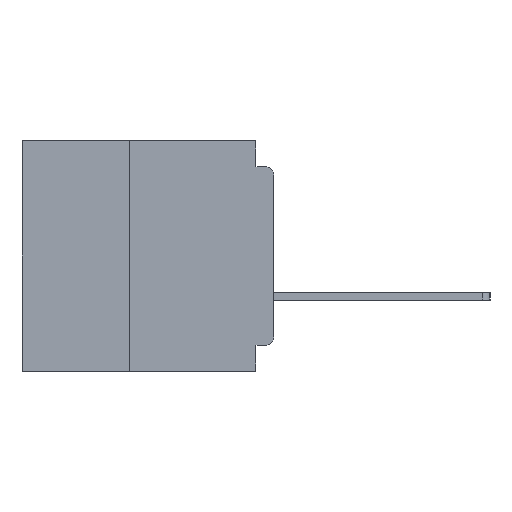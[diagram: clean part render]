
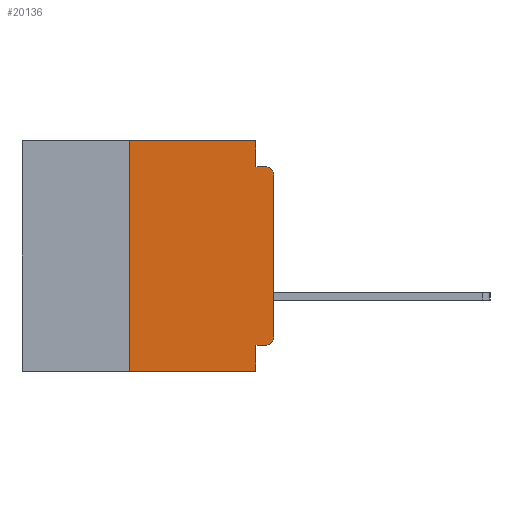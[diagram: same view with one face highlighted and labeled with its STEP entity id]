
A CAD part, left-side view. The second image highlights one B-rep face of the part: STEP entity #20136.
In plain terms, the highlighted planar face has unit normal (-1, 0, 0).
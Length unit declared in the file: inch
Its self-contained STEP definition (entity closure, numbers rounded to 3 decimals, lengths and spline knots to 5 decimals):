
#938 = ORIENTED_EDGE ( 'NONE', *, *, #48348, .F. ) ;
#1005 = VECTOR ( 'NONE', #35421, 39.37008 ) ;
#1330 = CARTESIAN_POINT ( 'NONE',  ( 0., 0.25, -0.4 ) ) ;
#1773 = VECTOR ( 'NONE', #25960, 39.37008 ) ;
#2149 = CIRCLE ( 'NONE', #40558, 0.015 ) ;
#2288 = DIRECTION ( 'NONE',  ( 0., -1., 0. ) ) ;
#2367 = VECTOR ( 'NONE', #25883, 39.37008 ) ;
#3299 = CARTESIAN_POINT ( 'NONE',  ( 0., 0.015, -0.045 ) ) ;
#5212 = ORIENTED_EDGE ( 'NONE', *, *, #49112, .T. ) ;
#5920 = VERTEX_POINT ( 'NONE', #15043 ) ;
#6289 = CARTESIAN_POINT ( 'NONE',  ( 0., 0., -0.355 ) ) ;
#7400 = CARTESIAN_POINT ( 'NONE',  ( 0., 0.015, -0.06 ) ) ;
#7617 = ORIENTED_EDGE ( 'NONE', *, *, #35024, .T. ) ;
#8090 = CARTESIAN_POINT ( 'NONE',  ( 0., 0.031, -0.355 ) ) ;
#8459 = VECTOR ( 'NONE', #44813, 39.37008 ) ;
#8874 = CARTESIAN_POINT ( 'NONE',  ( 0., 0.015, -0.34 ) ) ;
#9425 = VERTEX_POINT ( 'NONE', #21818 ) ;
#9551 = CARTESIAN_POINT ( 'NONE',  ( 0., 0.437, -0.4 ) ) ;
#10099 = CARTESIAN_POINT ( 'NONE',  ( 0., 0.437, 0. ) ) ;
#10802 = VECTOR ( 'NONE', #46721, 39.37008 ) ;
#11358 = DIRECTION ( 'NONE',  ( 0., 0., -1. ) ) ;
#11431 = LINE ( 'NONE', #39141, #1005 ) ;
#11525 = CARTESIAN_POINT ( 'NONE',  ( 0., 0.031, -0.4 ) ) ;
#12788 = CARTESIAN_POINT ( 'NONE',  ( 0., 0.031, 0. ) ) ;
#12807 = LINE ( 'NONE', #37500, #2367 ) ;
#12830 = DIRECTION ( 'NONE',  ( 0., 0., -1. ) ) ;
#14056 = DIRECTION ( 'NONE',  ( 0., 0., -1. ) ) ;
#15043 = CARTESIAN_POINT ( 'NONE',  ( 0., 0.031, -0.4 ) ) ;
#15621 = CIRCLE ( 'NONE', #40229, 0.015 ) ;
#17240 = CARTESIAN_POINT ( 'NONE',  ( 0., 0., -0.06 ) ) ;
#18258 = VECTOR ( 'NONE', #2288, 39.37008 ) ;
#20136 = ADVANCED_FACE ( 'NONE', ( #43924 ), #21844, .F. ) ;
#21818 = CARTESIAN_POINT ( 'NONE',  ( 0., 0., -0.34 ) ) ;
#21844 = PLANE ( 'NONE',  #34259 ) ;
#22664 = ORIENTED_EDGE ( 'NONE', *, *, #24728, .T. ) ;
#24728 = EDGE_CURVE ( 'NONE', #9425, #39866, #12807, .T. ) ;
#25067 = VERTEX_POINT ( 'NONE', #8090 ) ;
#25883 = DIRECTION ( 'NONE',  ( 0., 0., 1. ) ) ;
#25960 = DIRECTION ( 'NONE',  ( 0., 1., 0. ) ) ;
#26120 = VERTEX_POINT ( 'NONE', #27744 ) ;
#27744 = CARTESIAN_POINT ( 'NONE',  ( 0., 0.015, -0.355 ) ) ;
#27776 = VERTEX_POINT ( 'NONE', #3299 ) ;
#29022 = EDGE_LOOP ( 'NONE', ( #22664, #7617, #35274, #938, #48292, #48189, #39852, #42467, #47463, #5212 ) ) ;
#30227 = EDGE_CURVE ( 'NONE', #25067, #5920, #31806, .T. ) ;
#31806 = LINE ( 'NONE', #11525, #10802 ) ;
#33014 = VERTEX_POINT ( 'NONE', #48003 ) ;
#33109 = EDGE_CURVE ( 'NONE', #34341, #5920, #48802, .T. ) ;
#33227 = VERTEX_POINT ( 'NONE', #49159 ) ;
#33887 = VERTEX_POINT ( 'NONE', #45745 ) ;
#34259 = AXIS2_PLACEMENT_3D ( 'NONE', #10099, #37586, #14056 ) ;
#34341 = VERTEX_POINT ( 'NONE', #49066 ) ;
#34957 = DIRECTION ( 'NONE',  ( -1., 0., 0. ) ) ;
#35024 = EDGE_CURVE ( 'NONE', #39866, #27776, #15621, .T. ) ;
#35274 = ORIENTED_EDGE ( 'NONE', *, *, #47568, .F. ) ;
#35421 = DIRECTION ( 'NONE',  ( 0., -1., 0. ) ) ;
#36347 = DIRECTION ( 'NONE',  ( 0., 0., -1. ) ) ;
#36387 = DIRECTION ( 'NONE',  ( -1., 0., 0. ) ) ;
#36551 = DIRECTION ( 'NONE',  ( 0., 0., 1. ) ) ;
#37176 = VECTOR ( 'NONE', #36347, 39.37008 ) ;
#37500 = CARTESIAN_POINT ( 'NONE',  ( 0., 0., 0. ) ) ;
#37586 = DIRECTION ( 'NONE',  ( 1., 0., 0. ) ) ;
#39141 = CARTESIAN_POINT ( 'NONE',  ( 0., 0., -0.045 ) ) ;
#39852 = ORIENTED_EDGE ( 'NONE', *, *, #33109, .T. ) ;
#39866 = VERTEX_POINT ( 'NONE', #17240 ) ;
#40229 = AXIS2_PLACEMENT_3D ( 'NONE', #7400, #34957, #11358 ) ;
#40558 = AXIS2_PLACEMENT_3D ( 'NONE', #8874, #36387, #12830 ) ;
#41332 = VECTOR ( 'NONE', #36551, 39.37008 ) ;
#42467 = ORIENTED_EDGE ( 'NONE', *, *, #30227, .F. ) ;
#42546 = LINE ( 'NONE', #1330, #41332 ) ;
#43441 = LINE ( 'NONE', #6289, #1773 ) ;
#43655 = EDGE_CURVE ( 'NONE', #34341, #33227, #42546, .T. ) ;
#43924 = FACE_OUTER_BOUND ( 'NONE', #29022, .T. ) ;
#44813 = DIRECTION ( 'NONE',  ( 0., -1., 0. ) ) ;
#45745 = CARTESIAN_POINT ( 'NONE',  ( 0., 0.031, -0.045 ) ) ;
#46082 = EDGE_CURVE ( 'NONE', #26120, #25067, #43441, .T. ) ;
#46721 = DIRECTION ( 'NONE',  ( 0., 0., -1. ) ) ;
#47406 = LINE ( 'NONE', #12788, #37176 ) ;
#47463 = ORIENTED_EDGE ( 'NONE', *, *, #46082, .F. ) ;
#47568 = EDGE_CURVE ( 'NONE', #33887, #27776, #11431, .T. ) ;
#48003 = CARTESIAN_POINT ( 'NONE',  ( 0., 0.031, 0. ) ) ;
#48189 = ORIENTED_EDGE ( 'NONE', *, *, #43655, .F. ) ;
#48292 = ORIENTED_EDGE ( 'NONE', *, *, #49935, .F. ) ;
#48348 = EDGE_CURVE ( 'NONE', #33014, #33887, #47406, .T. ) ;
#48802 = LINE ( 'NONE', #9551, #8459 ) ;
#49066 = CARTESIAN_POINT ( 'NONE',  ( 0., 0.25, -0.4 ) ) ;
#49099 = CARTESIAN_POINT ( 'NONE',  ( 0., 0.437, 0. ) ) ;
#49112 = EDGE_CURVE ( 'NONE', #26120, #9425, #2149, .T. ) ;
#49159 = CARTESIAN_POINT ( 'NONE',  ( 0., 0.25, 0. ) ) ;
#49335 = LINE ( 'NONE', #49099, #18258 ) ;
#49935 = EDGE_CURVE ( 'NONE', #33227, #33014, #49335, .T. ) ;
